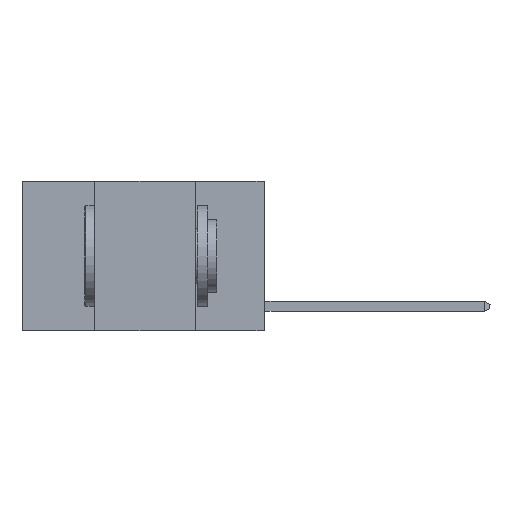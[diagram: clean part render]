
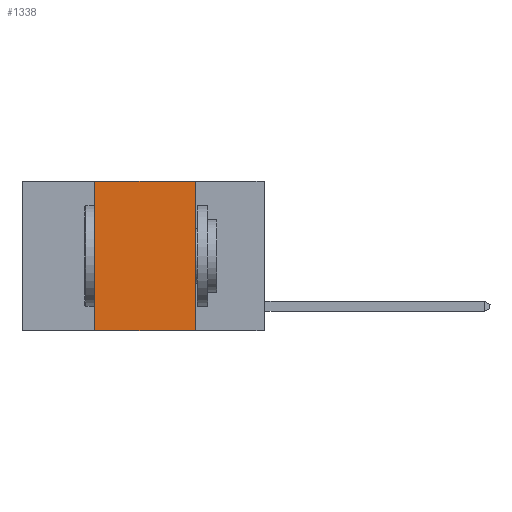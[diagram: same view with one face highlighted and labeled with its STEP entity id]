
A CAD part, left-side view. The second image highlights one B-rep face of the part: STEP entity #1338.
In plain terms, the highlighted planar face has unit normal (-1, 0, 0).
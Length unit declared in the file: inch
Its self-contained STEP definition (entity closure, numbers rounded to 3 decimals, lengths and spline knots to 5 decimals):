
#426 = CARTESIAN_POINT ( 'NONE',  ( 0., 0.17, 0. ) ) ;
#1338 = ADVANCED_FACE ( 'NONE', ( #16251 ), #10012, .F. ) ;
#1367 = DIRECTION ( 'NONE',  ( 0., 0., -1. ) ) ;
#1585 = VECTOR ( 'NONE', #2310, 39.37008 ) ;
#1785 = LINE ( 'NONE', #6292, #2546 ) ;
#2310 = DIRECTION ( 'NONE',  ( 0., -1., 0. ) ) ;
#2546 = VECTOR ( 'NONE', #8933, 39.37008 ) ;
#3197 = VERTEX_POINT ( 'NONE', #3349 ) ;
#3341 = ORIENTED_EDGE ( 'NONE', *, *, #15378, .T. ) ;
#3349 = CARTESIAN_POINT ( 'NONE',  ( 0., 0.17, -0.37 ) ) ;
#3367 = VECTOR ( 'NONE', #4048, 39.37008 ) ;
#3634 = ORIENTED_EDGE ( 'NONE', *, *, #11973, .F. ) ;
#3725 = LINE ( 'NONE', #17666, #1585 ) ;
#4048 = DIRECTION ( 'NONE',  ( 0., 0., -1. ) ) ;
#4518 = EDGE_CURVE ( 'NONE', #9821, #3197, #18420, .T. ) ;
#4692 = ORIENTED_EDGE ( 'NONE', *, *, #4518, .F. ) ;
#6292 = CARTESIAN_POINT ( 'NONE',  ( 0., 0.42, 0. ) ) ;
#8638 = VERTEX_POINT ( 'NONE', #16907 ) ;
#8692 = DIRECTION ( 'NONE',  ( 1., 0., 0. ) ) ;
#8768 = EDGE_LOOP ( 'NONE', ( #4692, #3634, #13229, #3341 ) ) ;
#8933 = DIRECTION ( 'NONE',  ( 0., 0., 1. ) ) ;
#9821 = VERTEX_POINT ( 'NONE', #426 ) ;
#9925 = CARTESIAN_POINT ( 'NONE',  ( 0., 0.42, 0. ) ) ;
#10012 = PLANE ( 'NONE',  #15666 ) ;
#10070 = VECTOR ( 'NONE', #17832, 39.37008 ) ;
#10672 = LINE ( 'NONE', #12091, #10070 ) ;
#11303 = CARTESIAN_POINT ( 'NONE',  ( 0., 0.6, 0. ) ) ;
#11973 = EDGE_CURVE ( 'NONE', #17621, #9821, #3725, .T. ) ;
#12091 = CARTESIAN_POINT ( 'NONE',  ( 0., 0.6, -0.37 ) ) ;
#13129 = CARTESIAN_POINT ( 'NONE',  ( 0., 0.17, 0. ) ) ;
#13229 = ORIENTED_EDGE ( 'NONE', *, *, #16064, .F. ) ;
#15378 = EDGE_CURVE ( 'NONE', #8638, #3197, #10672, .T. ) ;
#15666 = AXIS2_PLACEMENT_3D ( 'NONE', #11303, #8692, #1367 ) ;
#16064 = EDGE_CURVE ( 'NONE', #8638, #17621, #1785, .T. ) ;
#16251 = FACE_OUTER_BOUND ( 'NONE', #8768, .T. ) ;
#16907 = CARTESIAN_POINT ( 'NONE',  ( 0., 0.42, -0.37 ) ) ;
#17621 = VERTEX_POINT ( 'NONE', #9925 ) ;
#17666 = CARTESIAN_POINT ( 'NONE',  ( 0., 0.6, 0. ) ) ;
#17832 = DIRECTION ( 'NONE',  ( 0., -1., 0. ) ) ;
#18420 = LINE ( 'NONE', #13129, #3367 ) ;
